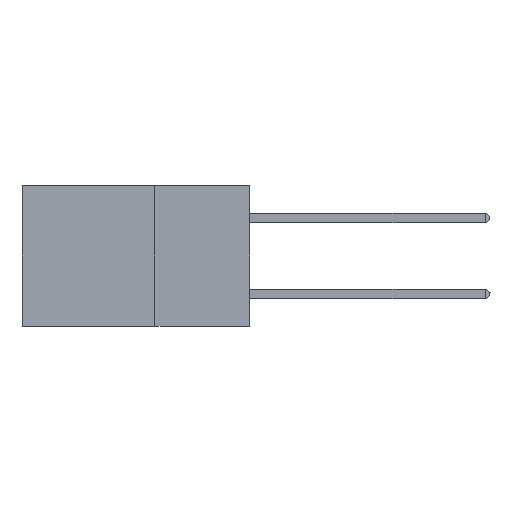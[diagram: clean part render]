
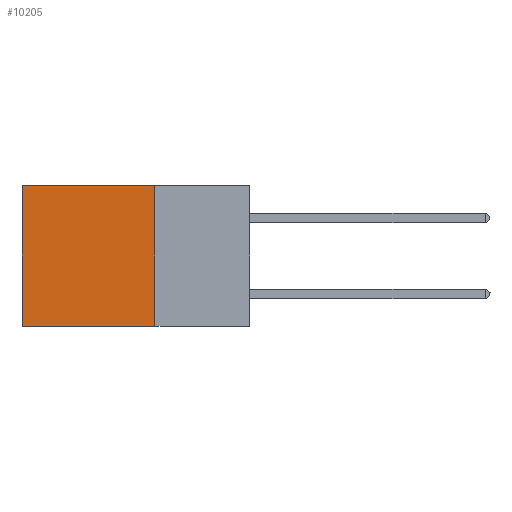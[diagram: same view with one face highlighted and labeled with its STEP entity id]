
A CAD part, left-side view. The second image highlights one B-rep face of the part: STEP entity #10205.
In plain terms, the highlighted planar face has unit normal (-1, 0, 0).
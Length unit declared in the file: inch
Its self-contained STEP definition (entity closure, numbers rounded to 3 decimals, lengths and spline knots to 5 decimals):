
#287 = CARTESIAN_POINT ( 'NONE',  ( 0.2875, 0.6, -0.37 ) ) ;
#1104 = VECTOR ( 'NONE', #12362, 39.37008 ) ;
#1423 = PLANE ( 'NONE',  #12194 ) ;
#3450 = DIRECTION ( 'NONE',  ( 0., 1., 0. ) ) ;
#6420 = EDGE_CURVE ( 'NONE', #12020, #7182, #7771, .T. ) ;
#6984 = FACE_OUTER_BOUND ( 'NONE', #8034, .T. ) ;
#7021 = DIRECTION ( 'NONE',  ( 0., 0., -1. ) ) ;
#7182 = VERTEX_POINT ( 'NONE', #287 ) ;
#7771 = LINE ( 'NONE', #10315, #1104 ) ;
#8034 = EDGE_LOOP ( 'NONE', ( #9008, #12064, #24037, #21554 ) ) ;
#8520 = VERTEX_POINT ( 'NONE', #22348 ) ;
#8570 = VERTEX_POINT ( 'NONE', #22435 ) ;
#8786 = EDGE_CURVE ( 'NONE', #8520, #7182, #8953, .T. ) ;
#8953 = LINE ( 'NONE', #22892, #24139 ) ;
#9008 = ORIENTED_EDGE ( 'NONE', *, *, #6420, .T. ) ;
#9574 = CARTESIAN_POINT ( 'NONE',  ( 0.2875, 0.25, 0. ) ) ;
#10205 = ADVANCED_FACE ( 'NONE', ( #6984 ), #1423, .F. ) ;
#10315 = CARTESIAN_POINT ( 'NONE',  ( 0.2875, 0.6, 0. ) ) ;
#11081 = DIRECTION ( 'NONE',  ( 0., 1., 0. ) ) ;
#11102 = CARTESIAN_POINT ( 'NONE',  ( 0.2875, 0.6, 0. ) ) ;
#11623 = DIRECTION ( 'NONE',  ( 0., 0., -1. ) ) ;
#12020 = VERTEX_POINT ( 'NONE', #11102 ) ;
#12064 = ORIENTED_EDGE ( 'NONE', *, *, #8786, .F. ) ;
#12194 = AXIS2_PLACEMENT_3D ( 'NONE', #9574, #23427, #11623 ) ;
#12362 = DIRECTION ( 'NONE',  ( 0., 0., -1. ) ) ;
#13357 = EDGE_CURVE ( 'NONE', #8570, #12020, #17540, .T. ) ;
#15233 = LINE ( 'NONE', #17057, #19199 ) ;
#17057 = CARTESIAN_POINT ( 'NONE',  ( 0.2875, 0.25, 0. ) ) ;
#17493 = CARTESIAN_POINT ( 'NONE',  ( 0.2875, 0.25, 0. ) ) ;
#17540 = LINE ( 'NONE', #17493, #25427 ) ;
#18857 = EDGE_CURVE ( 'NONE', #8570, #8520, #15233, .T. ) ;
#19199 = VECTOR ( 'NONE', #7021, 39.37008 ) ;
#21554 = ORIENTED_EDGE ( 'NONE', *, *, #13357, .T. ) ;
#22348 = CARTESIAN_POINT ( 'NONE',  ( 0.2875, 0.25, -0.37 ) ) ;
#22435 = CARTESIAN_POINT ( 'NONE',  ( 0.2875, 0.25, 0. ) ) ;
#22892 = CARTESIAN_POINT ( 'NONE',  ( 0.2875, 0.25, -0.37 ) ) ;
#23427 = DIRECTION ( 'NONE',  ( 1., 0., 0. ) ) ;
#24037 = ORIENTED_EDGE ( 'NONE', *, *, #18857, .F. ) ;
#24139 = VECTOR ( 'NONE', #11081, 39.37008 ) ;
#25427 = VECTOR ( 'NONE', #3450, 39.37008 ) ;
